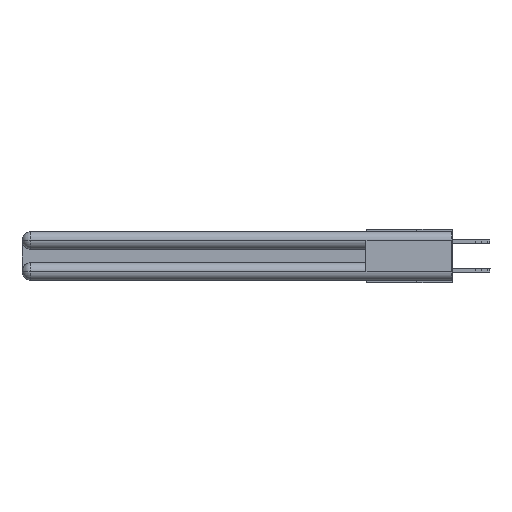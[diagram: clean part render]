
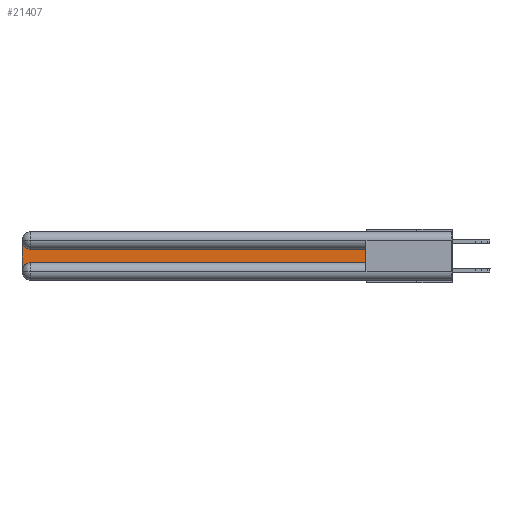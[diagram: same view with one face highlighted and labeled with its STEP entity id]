
A CAD part, left-side view. The second image highlights one B-rep face of the part: STEP entity #21407.
In plain terms, the highlighted planar face has unit normal (-1, 0, 0).
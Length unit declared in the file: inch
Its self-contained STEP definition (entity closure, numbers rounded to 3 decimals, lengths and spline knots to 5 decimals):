
#178 = LINE ( 'NONE', #22102, #9618 ) ;
#1016 = EDGE_CURVE ( 'NONE', #19326, #4636, #18809, .T. ) ;
#1097 = EDGE_LOOP ( 'NONE', ( #13660, #25586, #4629, #10057, #2807, #20542 ) ) ;
#1382 = DIRECTION ( 'NONE',  ( 0., 0., -1. ) ) ;
#1707 = CARTESIAN_POINT ( 'NONE',  ( 0.075, 3., -0.2775 ) ) ;
#2807 = ORIENTED_EDGE ( 'NONE', *, *, #16881, .T. ) ;
#3232 = CARTESIAN_POINT ( 'NONE',  ( 0.075, 3., -0.2175 ) ) ;
#3238 = LINE ( 'NONE', #19624, #10709 ) ;
#3398 = DIRECTION ( 'NONE',  ( 1., 0., 0. ) ) ;
#4045 = VERTEX_POINT ( 'NONE', #1707 ) ;
#4062 = VECTOR ( 'NONE', #19858, 39.37008 ) ;
#4629 = ORIENTED_EDGE ( 'NONE', *, *, #17433, .T. ) ;
#4636 = VERTEX_POINT ( 'NONE', #16064 ) ;
#4923 = CARTESIAN_POINT ( 'NONE',  ( 0.075, 0.6, -0.2175 ) ) ;
#5618 = DIRECTION ( 'NONE',  ( 0., -1., 0. ) ) ;
#6768 = DIRECTION ( 'NONE',  ( 0., 1., 0. ) ) ;
#7792 = VERTEX_POINT ( 'NONE', #21946 ) ;
#9254 = LINE ( 'NONE', #3232, #4062 ) ;
#9598 = DIRECTION ( 'NONE',  ( 0., 0., -1. ) ) ;
#9618 = VECTOR ( 'NONE', #5618, 39.37008 ) ;
#9678 = CARTESIAN_POINT ( 'NONE',  ( 0.075, 2.94, -0.0625 ) ) ;
#10057 = ORIENTED_EDGE ( 'NONE', *, *, #22707, .T. ) ;
#10122 = AXIS2_PLACEMENT_3D ( 'NONE', #13913, #16006, #9598 ) ;
#10671 = EDGE_CURVE ( 'NONE', #20608, #12819, #3238, .T. ) ;
#10709 = VECTOR ( 'NONE', #17657, 39.37008 ) ;
#11456 = AXIS2_PLACEMENT_3D ( 'NONE', #9678, #24146, #24060 ) ;
#12819 = VERTEX_POINT ( 'NONE', #14348 ) ;
#13660 = ORIENTED_EDGE ( 'NONE', *, *, #15883, .T. ) ;
#13913 = CARTESIAN_POINT ( 'NONE',  ( 0.075, 2.94, -0.2775 ) ) ;
#14348 = CARTESIAN_POINT ( 'NONE',  ( 0.075, 0.6, -0.1225 ) ) ;
#14544 = FACE_OUTER_BOUND ( 'NONE', #1097, .T. ) ;
#15883 = EDGE_CURVE ( 'NONE', #12819, #19326, #20438, .T. ) ;
#15924 = VECTOR ( 'NONE', #6768, 39.37008 ) ;
#16006 = DIRECTION ( 'NONE',  ( 1., 0., 0. ) ) ;
#16064 = CARTESIAN_POINT ( 'NONE',  ( 0.075, 3., -0.0625 ) ) ;
#16881 = EDGE_CURVE ( 'NONE', #7792, #20608, #178, .T. ) ;
#17087 = CARTESIAN_POINT ( 'NONE',  ( 0.075, 0.6, -0.1225 ) ) ;
#17433 = EDGE_CURVE ( 'NONE', #4636, #4045, #9254, .T. ) ;
#17657 = DIRECTION ( 'NONE',  ( 0., 0., 1. ) ) ;
#17964 = CARTESIAN_POINT ( 'NONE',  ( 0.075, 3., -0.1225 ) ) ;
#18809 = CIRCLE ( 'NONE', #11456, 0.06 ) ;
#19326 = VERTEX_POINT ( 'NONE', #20100 ) ;
#19624 = CARTESIAN_POINT ( 'NONE',  ( 0.075, 0.6, -0.2175 ) ) ;
#19858 = DIRECTION ( 'NONE',  ( 0., 0., -1. ) ) ;
#20100 = CARTESIAN_POINT ( 'NONE',  ( 0.075, 2.94, -0.1225 ) ) ;
#20438 = LINE ( 'NONE', #17087, #15924 ) ;
#20542 = ORIENTED_EDGE ( 'NONE', *, *, #10671, .T. ) ;
#20608 = VERTEX_POINT ( 'NONE', #4923 ) ;
#21407 = ADVANCED_FACE ( 'NONE', ( #14544 ), #22051, .F. ) ;
#21437 = CIRCLE ( 'NONE', #10122, 0.06 ) ;
#21946 = CARTESIAN_POINT ( 'NONE',  ( 0.075, 2.94, -0.2175 ) ) ;
#22051 = PLANE ( 'NONE',  #25455 ) ;
#22102 = CARTESIAN_POINT ( 'NONE',  ( 0.075, 0.6, -0.2175 ) ) ;
#22707 = EDGE_CURVE ( 'NONE', #4045, #7792, #21437, .T. ) ;
#24060 = DIRECTION ( 'NONE',  ( 0., 0., -1. ) ) ;
#24146 = DIRECTION ( 'NONE',  ( 1., 0., 0. ) ) ;
#25455 = AXIS2_PLACEMENT_3D ( 'NONE', #17964, #3398, #1382 ) ;
#25586 = ORIENTED_EDGE ( 'NONE', *, *, #1016, .T. ) ;
